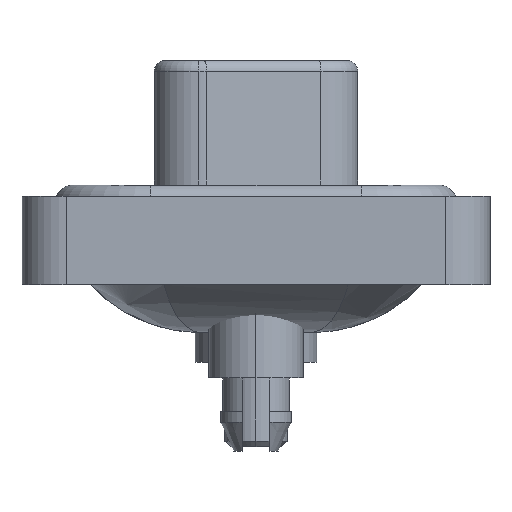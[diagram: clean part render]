
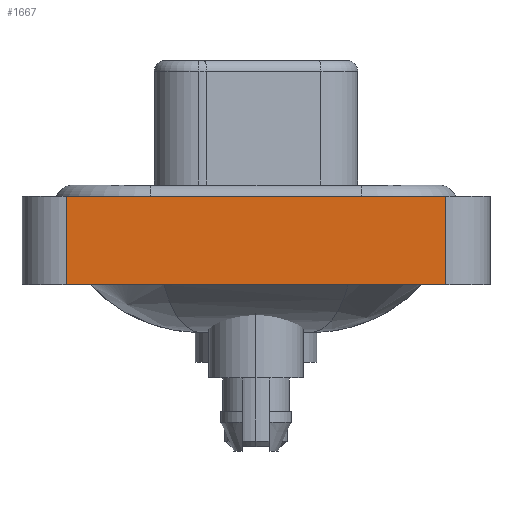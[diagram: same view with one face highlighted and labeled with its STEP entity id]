
A CAD part, left-side view. The second image highlights one B-rep face of the part: STEP entity #1667.
In plain terms, the highlighted planar face has unit normal (-1, 0, 0).
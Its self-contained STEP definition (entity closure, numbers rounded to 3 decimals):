
#321 = VECTOR ( 'NONE', #10409, 1000. ) ;
#751 = VERTEX_POINT ( 'NONE', #5224 ) ;
#1443 = CARTESIAN_POINT ( 'NONE',  ( -7.3, 8.55, 0.4 ) ) ;
#1630 = CARTESIAN_POINT ( 'NONE',  ( -7.3, -8.55, -3.6 ) ) ;
#1667 = ADVANCED_FACE ( 'NONE', ( #5727 ), #10117, .T. ) ;
#1975 = LINE ( 'NONE', #3542, #13008 ) ;
#2138 = DIRECTION ( 'NONE',  ( 0., 0., 1. ) ) ;
#2403 = DIRECTION ( 'NONE',  ( 0., 0., 1. ) ) ;
#3075 = ORIENTED_EDGE ( 'NONE', *, *, #15048, .F. ) ;
#3542 = CARTESIAN_POINT ( 'NONE',  ( -7.3, 8.55, -3.6 ) ) ;
#4375 = ORIENTED_EDGE ( 'NONE', *, *, #6422, .T. ) ;
#4919 = DIRECTION ( 'NONE',  ( -1., 0., 0. ) ) ;
#5208 = VECTOR ( 'NONE', #2403, 1000. ) ;
#5216 = EDGE_CURVE ( 'NONE', #16791, #14609, #1975, .T. ) ;
#5224 = CARTESIAN_POINT ( 'NONE',  ( -7.3, -8.55, 0.4 ) ) ;
#5727 = FACE_OUTER_BOUND ( 'NONE', #12755, .T. ) ;
#6422 = EDGE_CURVE ( 'NONE', #10224, #751, #10227, .T. ) ;
#7265 = VECTOR ( 'NONE', #7926, 1000. ) ;
#7566 = DIRECTION ( 'NONE',  ( 0., 0., 1. ) ) ;
#7651 = LINE ( 'NONE', #14576, #7265 ) ;
#7926 = DIRECTION ( 'NONE',  ( 0., -1., 0. ) ) ;
#8323 = CARTESIAN_POINT ( 'NONE',  ( -7.3, 8.55, -3.6 ) ) ;
#9194 = LINE ( 'NONE', #11719, #321 ) ;
#9730 = AXIS2_PLACEMENT_3D ( 'NONE', #12746, #4919, #2138 ) ;
#10117 = PLANE ( 'NONE',  #9730 ) ;
#10224 = VERTEX_POINT ( 'NONE', #1630 ) ;
#10227 = LINE ( 'NONE', #14246, #5208 ) ;
#10409 = DIRECTION ( 'NONE',  ( 0., -1., 0. ) ) ;
#11719 = CARTESIAN_POINT ( 'NONE',  ( -7.3, -8.55, -3.6 ) ) ;
#12746 = CARTESIAN_POINT ( 'NONE',  ( -7.3, -8.55, -3.6 ) ) ;
#12755 = EDGE_LOOP ( 'NONE', ( #4375, #3075, #16961, #15838 ) ) ;
#13008 = VECTOR ( 'NONE', #7566, 1000. ) ;
#14246 = CARTESIAN_POINT ( 'NONE',  ( -7.3, -8.55, -3.6 ) ) ;
#14576 = CARTESIAN_POINT ( 'NONE',  ( -7.3, -8.55, 0.4 ) ) ;
#14609 = VERTEX_POINT ( 'NONE', #1443 ) ;
#15048 = EDGE_CURVE ( 'NONE', #14609, #751, #7651, .T. ) ;
#15838 = ORIENTED_EDGE ( 'NONE', *, *, #17257, .T. ) ;
#16791 = VERTEX_POINT ( 'NONE', #8323 ) ;
#16961 = ORIENTED_EDGE ( 'NONE', *, *, #5216, .F. ) ;
#17257 = EDGE_CURVE ( 'NONE', #16791, #10224, #9194, .T. ) ;
